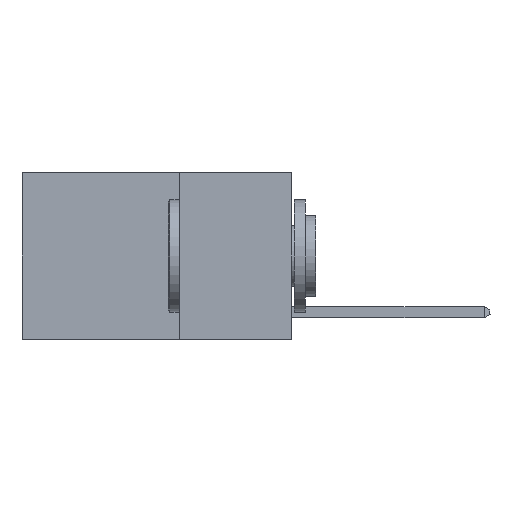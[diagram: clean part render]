
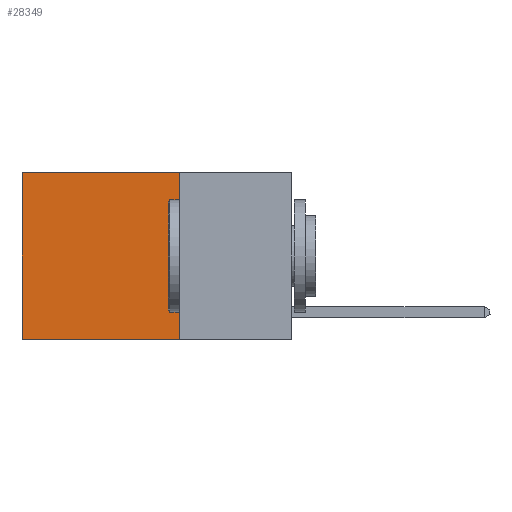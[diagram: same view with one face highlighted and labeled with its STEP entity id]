
A CAD part, left-side view. The second image highlights one B-rep face of the part: STEP entity #28349.
In plain terms, the highlighted planar face has unit normal (-1, 0, 0).
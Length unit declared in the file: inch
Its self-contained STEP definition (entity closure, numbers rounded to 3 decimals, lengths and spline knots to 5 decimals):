
#1152 = LINE ( 'NONE', #18787, #8730 ) ;
#1226 = CARTESIAN_POINT ( 'NONE',  ( 0.2625, 0.6, 0. ) ) ;
#1239 = EDGE_CURVE ( 'NONE', #11141, #11758, #14179, .T. ) ;
#3489 = ORIENTED_EDGE ( 'NONE', *, *, #1239, .F. ) ;
#4305 = EDGE_CURVE ( 'NONE', #19818, #19132, #13646, .T. ) ;
#4981 = AXIS2_PLACEMENT_3D ( 'NONE', #19055, #10356, #23984 ) ;
#7399 = LINE ( 'NONE', #24755, #25375 ) ;
#7411 = EDGE_LOOP ( 'NONE', ( #19173, #3489, #27269, #21362 ) ) ;
#8730 = VECTOR ( 'NONE', #27660, 39.37008 ) ;
#8964 = CARTESIAN_POINT ( 'NONE',  ( 0.2625, 0.25, -0.37 ) ) ;
#10221 = PLANE ( 'NONE',  #4981 ) ;
#10356 = DIRECTION ( 'NONE',  ( 1., 0., 0. ) ) ;
#11141 = VERTEX_POINT ( 'NONE', #8964 ) ;
#11758 = VERTEX_POINT ( 'NONE', #15233 ) ;
#13646 = LINE ( 'NONE', #28611, #24144 ) ;
#14179 = LINE ( 'NONE', #23062, #22199 ) ;
#15233 = CARTESIAN_POINT ( 'NONE',  ( 0.2625, 0.6, -0.37 ) ) ;
#15251 = EDGE_CURVE ( 'NONE', #19132, #11758, #7399, .T. ) ;
#16122 = EDGE_CURVE ( 'NONE', #19818, #11141, #1152, .T. ) ;
#16178 = DIRECTION ( 'NONE',  ( 0., 0., -1. ) ) ;
#16856 = FACE_OUTER_BOUND ( 'NONE', #7411, .T. ) ;
#17542 = CARTESIAN_POINT ( 'NONE',  ( 0.2625, 0.25, 0. ) ) ;
#18787 = CARTESIAN_POINT ( 'NONE',  ( 0.2625, 0.25, 0. ) ) ;
#19055 = CARTESIAN_POINT ( 'NONE',  ( 0.2625, 0.25, 0. ) ) ;
#19132 = VERTEX_POINT ( 'NONE', #1226 ) ;
#19173 = ORIENTED_EDGE ( 'NONE', *, *, #15251, .T. ) ;
#19818 = VERTEX_POINT ( 'NONE', #17542 ) ;
#21362 = ORIENTED_EDGE ( 'NONE', *, *, #4305, .T. ) ;
#22199 = VECTOR ( 'NONE', #25658, 39.37008 ) ;
#22360 = DIRECTION ( 'NONE',  ( 0., 1., 0. ) ) ;
#23062 = CARTESIAN_POINT ( 'NONE',  ( 0.2625, 0.25, -0.37 ) ) ;
#23984 = DIRECTION ( 'NONE',  ( 0., 0., -1. ) ) ;
#24144 = VECTOR ( 'NONE', #22360, 39.37008 ) ;
#24755 = CARTESIAN_POINT ( 'NONE',  ( 0.2625, 0.6, 0. ) ) ;
#25375 = VECTOR ( 'NONE', #16178, 39.37008 ) ;
#25658 = DIRECTION ( 'NONE',  ( 0., 1., 0. ) ) ;
#27269 = ORIENTED_EDGE ( 'NONE', *, *, #16122, .F. ) ;
#27660 = DIRECTION ( 'NONE',  ( 0., 0., -1. ) ) ;
#28349 = ADVANCED_FACE ( 'NONE', ( #16856 ), #10221, .F. ) ;
#28611 = CARTESIAN_POINT ( 'NONE',  ( 0.2625, 0.25, 0. ) ) ;
